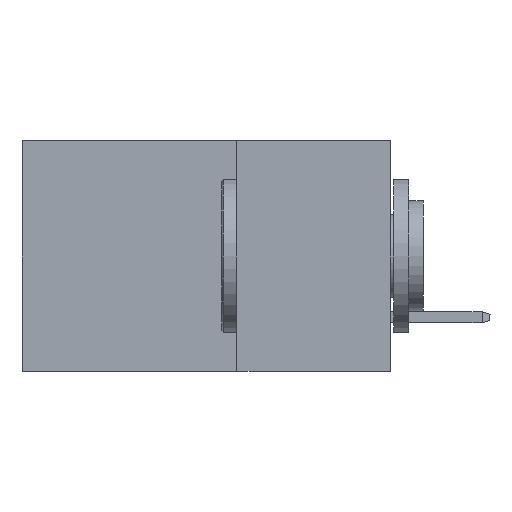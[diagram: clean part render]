
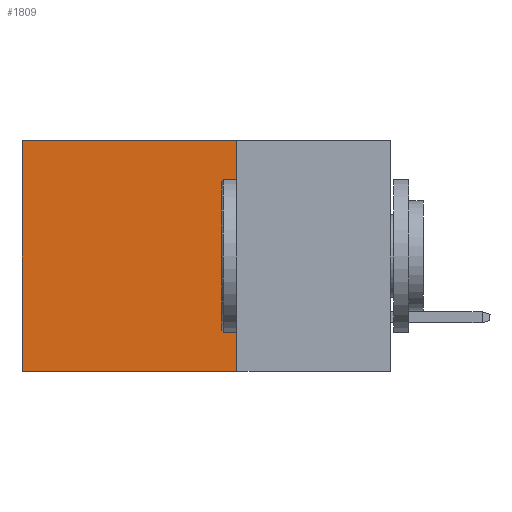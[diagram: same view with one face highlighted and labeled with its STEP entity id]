
A CAD part, left-side view. The second image highlights one B-rep face of the part: STEP entity #1809.
In plain terms, the highlighted planar face has unit normal (-1, 0, 0).
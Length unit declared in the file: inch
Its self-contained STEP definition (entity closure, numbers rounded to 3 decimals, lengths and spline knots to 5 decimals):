
#363 = CARTESIAN_POINT ( 'NONE',  ( 0.2875, 0.25, 0. ) ) ;
#696 = DIRECTION ( 'NONE',  ( 1., 0., 0. ) ) ;
#1544 = CARTESIAN_POINT ( 'NONE',  ( 0.2875, 0.25, 0. ) ) ;
#1730 = CARTESIAN_POINT ( 'NONE',  ( 0.2875, 0.25, -0.375 ) ) ;
#1809 = ADVANCED_FACE ( 'NONE', ( #2853 ), #5881, .F. ) ;
#1969 = VECTOR ( 'NONE', #10851, 39.37008 ) ;
#2199 = CARTESIAN_POINT ( 'NONE',  ( 0.2875, 0.6, -0.375 ) ) ;
#2453 = VECTOR ( 'NONE', #5162, 39.37008 ) ;
#2526 = EDGE_CURVE ( 'NONE', #4030, #7266, #10429, .T. ) ;
#2528 = LINE ( 'NONE', #363, #5359 ) ;
#2721 = DIRECTION ( 'NONE',  ( 0., 1., 0. ) ) ;
#2853 = FACE_OUTER_BOUND ( 'NONE', #10869, .T. ) ;
#3383 = VERTEX_POINT ( 'NONE', #2199 ) ;
#4030 = VERTEX_POINT ( 'NONE', #1544 ) ;
#4965 = DIRECTION ( 'NONE',  ( 0., 0., -1. ) ) ;
#5162 = DIRECTION ( 'NONE',  ( 0., 0., -1. ) ) ;
#5329 = EDGE_CURVE ( 'NONE', #7024, #3383, #13042, .T. ) ;
#5359 = VECTOR ( 'NONE', #2721, 39.37008 ) ;
#5881 = PLANE ( 'NONE',  #12602 ) ;
#6006 = EDGE_CURVE ( 'NONE', #7266, #3383, #11514, .T. ) ;
#6687 = CARTESIAN_POINT ( 'NONE',  ( 0.2875, 0.25, -0.375 ) ) ;
#7024 = VERTEX_POINT ( 'NONE', #8531 ) ;
#7266 = VERTEX_POINT ( 'NONE', #6687 ) ;
#8531 = CARTESIAN_POINT ( 'NONE',  ( 0.2875, 0.6, 0. ) ) ;
#8599 = ORIENTED_EDGE ( 'NONE', *, *, #2526, .F. ) ;
#9402 = DIRECTION ( 'NONE',  ( 0., 1., 0. ) ) ;
#10429 = LINE ( 'NONE', #13532, #2453 ) ;
#10450 = CARTESIAN_POINT ( 'NONE',  ( 0.2875, 0.25, -0.375 ) ) ;
#10851 = DIRECTION ( 'NONE',  ( 0., 0., -1. ) ) ;
#10869 = EDGE_LOOP ( 'NONE', ( #11415, #11912, #8599, #11043 ) ) ;
#11043 = ORIENTED_EDGE ( 'NONE', *, *, #12274, .T. ) ;
#11415 = ORIENTED_EDGE ( 'NONE', *, *, #5329, .T. ) ;
#11514 = LINE ( 'NONE', #10450, #12669 ) ;
#11906 = CARTESIAN_POINT ( 'NONE',  ( 0.2875, 0.6, -0.375 ) ) ;
#11912 = ORIENTED_EDGE ( 'NONE', *, *, #6006, .F. ) ;
#12274 = EDGE_CURVE ( 'NONE', #4030, #7024, #2528, .T. ) ;
#12602 = AXIS2_PLACEMENT_3D ( 'NONE', #1730, #696, #4965 ) ;
#12669 = VECTOR ( 'NONE', #9402, 39.37008 ) ;
#13042 = LINE ( 'NONE', #11906, #1969 ) ;
#13532 = CARTESIAN_POINT ( 'NONE',  ( 0.2875, 0.25, -0.375 ) ) ;
